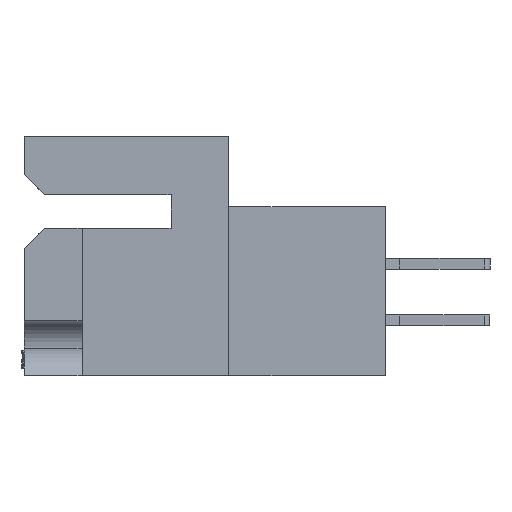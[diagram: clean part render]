
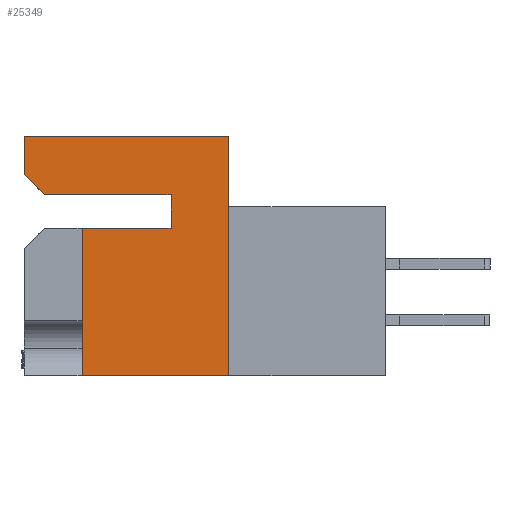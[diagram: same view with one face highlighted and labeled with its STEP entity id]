
A CAD part, left-side view. The second image highlights one B-rep face of the part: STEP entity #25349.
In plain terms, the highlighted planar face has unit normal (-1, 0, 0).
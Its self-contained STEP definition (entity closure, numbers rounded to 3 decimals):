
#53 = CARTESIAN_POINT ( 'NONE',  ( 0., 0., 0. ) ) ;
#527 = CARTESIAN_POINT ( 'NONE',  ( 0., 11.506, -2.159 ) ) ;
#661 = LINE ( 'NONE', #23318, #5312 ) ;
#692 = EDGE_CURVE ( 'NONE', #13756, #14055, #12428, .T. ) ;
#980 = EDGE_CURVE ( 'NONE', #20251, #5864, #27485, .T. ) ;
#1062 = PLANE ( 'NONE',  #12375 ) ;
#1876 = DIRECTION ( 'NONE',  ( 0., 0., 1. ) ) ;
#2600 = ORIENTED_EDGE ( 'NONE', *, *, #692, .F. ) ;
#2729 = LINE ( 'NONE', #53, #21729 ) ;
#4549 = DIRECTION ( 'NONE',  ( 0., -1., 0. ) ) ;
#5312 = VECTOR ( 'NONE', #18816, 1000. ) ;
#5675 = VERTEX_POINT ( 'NONE', #16326 ) ;
#5762 = EDGE_CURVE ( 'NONE', #14055, #7163, #7164, .T. ) ;
#5851 = DIRECTION ( 'NONE',  ( 0., 1., 0. ) ) ;
#5864 = VERTEX_POINT ( 'NONE', #18096 ) ;
#6208 = ORIENTED_EDGE ( 'NONE', *, *, #8965, .F. ) ;
#6290 = ORIENTED_EDGE ( 'NONE', *, *, #18712, .F. ) ;
#6299 = VECTOR ( 'NONE', #12128, 1000. ) ;
#6381 = DIRECTION ( 'NONE',  ( 0., -1., 0. ) ) ;
#6463 = VERTEX_POINT ( 'NONE', #16033 ) ;
#6992 = CARTESIAN_POINT ( 'NONE',  ( 0., 3.251, -3.302 ) ) ;
#7163 = VERTEX_POINT ( 'NONE', #16969 ) ;
#7164 = LINE ( 'NONE', #12697, #9665 ) ;
#8361 = CARTESIAN_POINT ( 'NONE',  ( 0., 10.363, -3.302 ) ) ;
#8785 = LINE ( 'NONE', #15631, #9168 ) ;
#8965 = EDGE_CURVE ( 'NONE', #5864, #13756, #8785, .T. ) ;
#9168 = VECTOR ( 'NONE', #6381, 1000. ) ;
#9665 = VECTOR ( 'NONE', #5851, 1000. ) ;
#10270 = CARTESIAN_POINT ( 'NONE',  ( 0., 3.251, -5.182 ) ) ;
#10696 = EDGE_CURVE ( 'NONE', #28696, #5675, #21313, .T. ) ;
#11090 = CARTESIAN_POINT ( 'NONE',  ( 0., 11.506, -13.487 ) ) ;
#12128 = DIRECTION ( 'NONE',  ( 0., 0., 1. ) ) ;
#12375 = AXIS2_PLACEMENT_3D ( 'NONE', #19322, #19043, #26258 ) ;
#12428 = LINE ( 'NONE', #14533, #6299 ) ;
#12697 = CARTESIAN_POINT ( 'NONE',  ( 0., 0., -3.302 ) ) ;
#13756 = VERTEX_POINT ( 'NONE', #10270 ) ;
#13905 = CARTESIAN_POINT ( 'NONE',  ( 0., 11.506, 0. ) ) ;
#14055 = VERTEX_POINT ( 'NONE', #6992 ) ;
#14533 = CARTESIAN_POINT ( 'NONE',  ( 0., 3.251, -5.182 ) ) ;
#15631 = CARTESIAN_POINT ( 'NONE',  ( 0., 0., -5.182 ) ) ;
#16033 = CARTESIAN_POINT ( 'NONE',  ( 0., 0., -13.487 ) ) ;
#16326 = CARTESIAN_POINT ( 'NONE',  ( 0., 0., 0. ) ) ;
#16368 = ORIENTED_EDGE ( 'NONE', *, *, #23211, .T. ) ;
#16488 = EDGE_CURVE ( 'NONE', #5675, #6463, #2729, .T. ) ;
#16969 = CARTESIAN_POINT ( 'NONE',  ( 0., 10.363, -3.302 ) ) ;
#17296 = EDGE_LOOP ( 'NONE', ( #26302, #29169, #23737, #6290, #16368, #28921, #2600, #6208, #23601 ) ) ;
#18096 = CARTESIAN_POINT ( 'NONE',  ( 0., 8.255, -5.182 ) ) ;
#18281 = VECTOR ( 'NONE', #29160, 1000. ) ;
#18712 = EDGE_CURVE ( 'NONE', #20099, #28696, #22094, .T. ) ;
#18720 = CARTESIAN_POINT ( 'NONE',  ( 0., 11.506, 0. ) ) ;
#18816 = DIRECTION ( 'NONE',  ( 0., 1., 0. ) ) ;
#19043 = DIRECTION ( 'NONE',  ( 1., 0., 0. ) ) ;
#19322 = CARTESIAN_POINT ( 'NONE',  ( 0., 0., 0. ) ) ;
#19887 = CARTESIAN_POINT ( 'NONE',  ( 0., 8.255, -13.487 ) ) ;
#20099 = VERTEX_POINT ( 'NONE', #527 ) ;
#20251 = VERTEX_POINT ( 'NONE', #19887 ) ;
#20336 = DIRECTION ( 'NONE',  ( 0., 0., -1. ) ) ;
#21313 = LINE ( 'NONE', #13905, #25260 ) ;
#21729 = VECTOR ( 'NONE', #20336, 1000. ) ;
#22094 = LINE ( 'NONE', #11090, #28917 ) ;
#22135 = FACE_OUTER_BOUND ( 'NONE', #17296, .T. ) ;
#23211 = EDGE_CURVE ( 'NONE', #20099, #7163, #24372, .T. ) ;
#23318 = CARTESIAN_POINT ( 'NONE',  ( 0., -8.814, -13.487 ) ) ;
#23601 = ORIENTED_EDGE ( 'NONE', *, *, #980, .F. ) ;
#23737 = ORIENTED_EDGE ( 'NONE', *, *, #10696, .F. ) ;
#24372 = LINE ( 'NONE', #8361, #18281 ) ;
#25260 = VECTOR ( 'NONE', #4549, 1000. ) ;
#25349 = ADVANCED_FACE ( 'NONE', ( #22135 ), #1062, .F. ) ;
#25663 = DIRECTION ( 'NONE',  ( 0., 0., 1. ) ) ;
#25682 = VECTOR ( 'NONE', #25663, 1000. ) ;
#25758 = CARTESIAN_POINT ( 'NONE',  ( 0., 8.255, -5.182 ) ) ;
#25962 = EDGE_CURVE ( 'NONE', #6463, #20251, #661, .T. ) ;
#26258 = DIRECTION ( 'NONE',  ( 0., 0., -1. ) ) ;
#26302 = ORIENTED_EDGE ( 'NONE', *, *, #25962, .F. ) ;
#27485 = LINE ( 'NONE', #25758, #25682 ) ;
#28696 = VERTEX_POINT ( 'NONE', #18720 ) ;
#28917 = VECTOR ( 'NONE', #1876, 1000. ) ;
#28921 = ORIENTED_EDGE ( 'NONE', *, *, #5762, .F. ) ;
#29160 = DIRECTION ( 'NONE',  ( 0., -0.707, -0.707 ) ) ;
#29169 = ORIENTED_EDGE ( 'NONE', *, *, #16488, .F. ) ;
